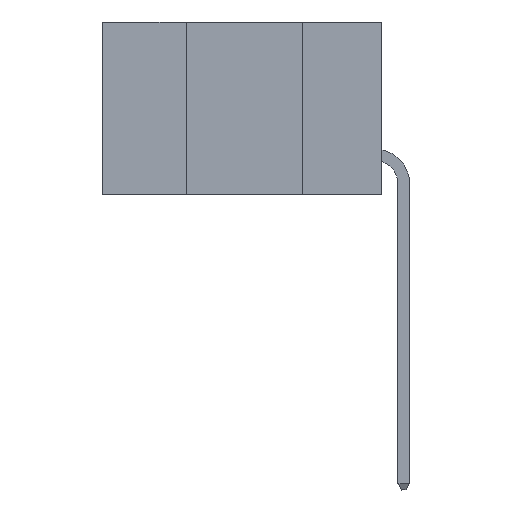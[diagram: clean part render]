
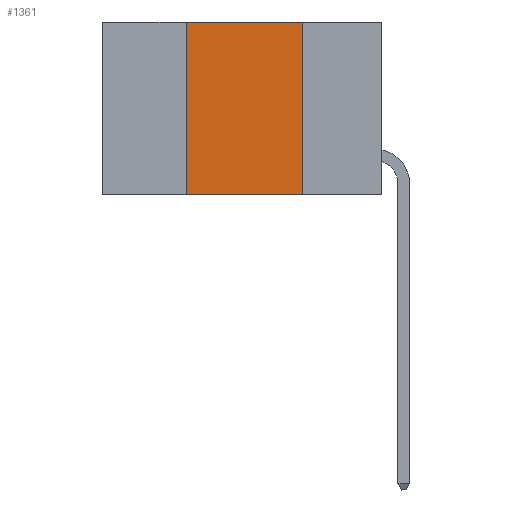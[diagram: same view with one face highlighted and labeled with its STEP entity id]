
A CAD part, left-side view. The second image highlights one B-rep face of the part: STEP entity #1361.
In plain terms, the highlighted planar face has unit normal (-1, 0, 0).
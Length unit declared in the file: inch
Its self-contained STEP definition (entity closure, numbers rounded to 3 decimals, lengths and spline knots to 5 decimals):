
#752 = EDGE_CURVE ( 'NONE', #13168, #17485, #10818, .T. ) ;
#974 = CARTESIAN_POINT ( 'NONE',  ( 0., 0.6, 0. ) ) ;
#1361 = ADVANCED_FACE ( 'NONE', ( #12903 ), #4402, .F. ) ;
#2883 = ORIENTED_EDGE ( 'NONE', *, *, #7879, .F. ) ;
#3080 = ORIENTED_EDGE ( 'NONE', *, *, #19282, .T. ) ;
#3949 = DIRECTION ( 'NONE',  ( 0., -1., 0. ) ) ;
#4402 = PLANE ( 'NONE',  #12169 ) ;
#4441 = LINE ( 'NONE', #15548, #7071 ) ;
#4477 = LINE ( 'NONE', #5097, #16750 ) ;
#5097 = CARTESIAN_POINT ( 'NONE',  ( 0., 0.17, 0. ) ) ;
#5627 = CARTESIAN_POINT ( 'NONE',  ( 0., 0.6, -0.37 ) ) ;
#5683 = EDGE_LOOP ( 'NONE', ( #15937, #13250, #2883, #3080 ) ) ;
#5966 = DIRECTION ( 'NONE',  ( 0., -1., 0. ) ) ;
#6339 = VECTOR ( 'NONE', #3949, 39.37008 ) ;
#7071 = VECTOR ( 'NONE', #7181, 39.37008 ) ;
#7181 = DIRECTION ( 'NONE',  ( 0., 0., 1. ) ) ;
#7475 = VECTOR ( 'NONE', #5966, 39.37008 ) ;
#7819 = CARTESIAN_POINT ( 'NONE',  ( 0., 0.42, -0.37 ) ) ;
#7879 = EDGE_CURVE ( 'NONE', #15115, #13168, #4441, .T. ) ;
#10818 = LINE ( 'NONE', #974, #6339 ) ;
#10997 = CARTESIAN_POINT ( 'NONE',  ( 0., 0.17, -0.37 ) ) ;
#12169 = AXIS2_PLACEMENT_3D ( 'NONE', #16677, #12272, #17141 ) ;
#12272 = DIRECTION ( 'NONE',  ( 1., 0., 0. ) ) ;
#12903 = FACE_OUTER_BOUND ( 'NONE', #5683, .T. ) ;
#13137 = VERTEX_POINT ( 'NONE', #10997 ) ;
#13168 = VERTEX_POINT ( 'NONE', #19046 ) ;
#13250 = ORIENTED_EDGE ( 'NONE', *, *, #752, .F. ) ;
#14507 = LINE ( 'NONE', #5627, #7475 ) ;
#15115 = VERTEX_POINT ( 'NONE', #7819 ) ;
#15548 = CARTESIAN_POINT ( 'NONE',  ( 0., 0.42, 0. ) ) ;
#15937 = ORIENTED_EDGE ( 'NONE', *, *, #16967, .F. ) ;
#16677 = CARTESIAN_POINT ( 'NONE',  ( 0., 0.6, 0. ) ) ;
#16750 = VECTOR ( 'NONE', #17170, 39.37008 ) ;
#16967 = EDGE_CURVE ( 'NONE', #17485, #13137, #4477, .T. ) ;
#17141 = DIRECTION ( 'NONE',  ( 0., 0., -1. ) ) ;
#17170 = DIRECTION ( 'NONE',  ( 0., 0., -1. ) ) ;
#17485 = VERTEX_POINT ( 'NONE', #19089 ) ;
#19046 = CARTESIAN_POINT ( 'NONE',  ( 0., 0.42, 0. ) ) ;
#19089 = CARTESIAN_POINT ( 'NONE',  ( 0., 0.17, 0. ) ) ;
#19282 = EDGE_CURVE ( 'NONE', #15115, #13137, #14507, .T. ) ;
